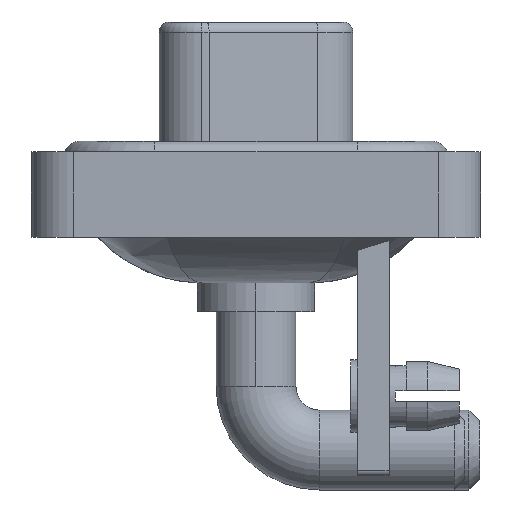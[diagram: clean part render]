
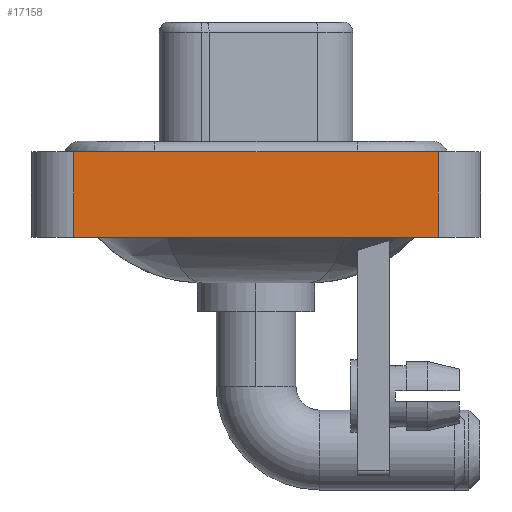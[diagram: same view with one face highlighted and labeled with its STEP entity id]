
A CAD part, left-side view. The second image highlights one B-rep face of the part: STEP entity #17158.
In plain terms, the highlighted planar face has unit normal (-1, 0, 0).
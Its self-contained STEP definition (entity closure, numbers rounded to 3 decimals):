
#466 = DIRECTION ( 'NONE',  ( 0., 0., 1. ) ) ;
#1835 = LINE ( 'NONE', #8472, #16503 ) ;
#2279 = DIRECTION ( 'NONE',  ( -1., 0., 0. ) ) ;
#2525 = CARTESIAN_POINT ( 'NONE',  ( -7.3, 8.55, -3.6 ) ) ;
#3016 = EDGE_CURVE ( 'NONE', #9323, #13770, #9100, .T. ) ;
#4054 = VERTEX_POINT ( 'NONE', #5551 ) ;
#4618 = ORIENTED_EDGE ( 'NONE', *, *, #18474, .F. ) ;
#5551 = CARTESIAN_POINT ( 'NONE',  ( -7.3, 8.55, 0.4 ) ) ;
#5718 = EDGE_CURVE ( 'NONE', #13770, #14948, #12703, .T. ) ;
#7108 = LINE ( 'NONE', #18781, #16730 ) ;
#7757 = ORIENTED_EDGE ( 'NONE', *, *, #5718, .T. ) ;
#8331 = EDGE_CURVE ( 'NONE', #4054, #14948, #1835, .T. ) ;
#8472 = CARTESIAN_POINT ( 'NONE',  ( -7.3, -8.55, 0.4 ) ) ;
#9100 = LINE ( 'NONE', #12422, #19740 ) ;
#9268 = DIRECTION ( 'NONE',  ( 0., 0., 1. ) ) ;
#9323 = VERTEX_POINT ( 'NONE', #2525 ) ;
#10348 = AXIS2_PLACEMENT_3D ( 'NONE', #12358, #2279, #17412 ) ;
#11791 = ORIENTED_EDGE ( 'NONE', *, *, #8331, .F. ) ;
#12358 = CARTESIAN_POINT ( 'NONE',  ( -7.3, -8.55, -3.6 ) ) ;
#12422 = CARTESIAN_POINT ( 'NONE',  ( -7.3, -8.55, -3.6 ) ) ;
#12703 = LINE ( 'NONE', #19405, #16755 ) ;
#13013 = CARTESIAN_POINT ( 'NONE',  ( -7.3, -8.55, 0.4 ) ) ;
#13343 = CARTESIAN_POINT ( 'NONE',  ( -7.3, -8.55, -3.6 ) ) ;
#13770 = VERTEX_POINT ( 'NONE', #13343 ) ;
#13942 = DIRECTION ( 'NONE',  ( 0., -1., 0. ) ) ;
#14948 = VERTEX_POINT ( 'NONE', #13013 ) ;
#14962 = DIRECTION ( 'NONE',  ( 0., -1., 0. ) ) ;
#16503 = VECTOR ( 'NONE', #14962, 1000. ) ;
#16509 = ORIENTED_EDGE ( 'NONE', *, *, #3016, .T. ) ;
#16730 = VECTOR ( 'NONE', #466, 1000. ) ;
#16755 = VECTOR ( 'NONE', #9268, 1000. ) ;
#17158 = ADVANCED_FACE ( 'NONE', ( #20925 ), #20812, .T. ) ;
#17412 = DIRECTION ( 'NONE',  ( 0., 0., 1. ) ) ;
#18471 = EDGE_LOOP ( 'NONE', ( #7757, #11791, #4618, #16509 ) ) ;
#18474 = EDGE_CURVE ( 'NONE', #9323, #4054, #7108, .T. ) ;
#18781 = CARTESIAN_POINT ( 'NONE',  ( -7.3, 8.55, -3.6 ) ) ;
#19405 = CARTESIAN_POINT ( 'NONE',  ( -7.3, -8.55, -3.6 ) ) ;
#19740 = VECTOR ( 'NONE', #13942, 1000. ) ;
#20812 = PLANE ( 'NONE',  #10348 ) ;
#20925 = FACE_OUTER_BOUND ( 'NONE', #18471, .T. ) ;
